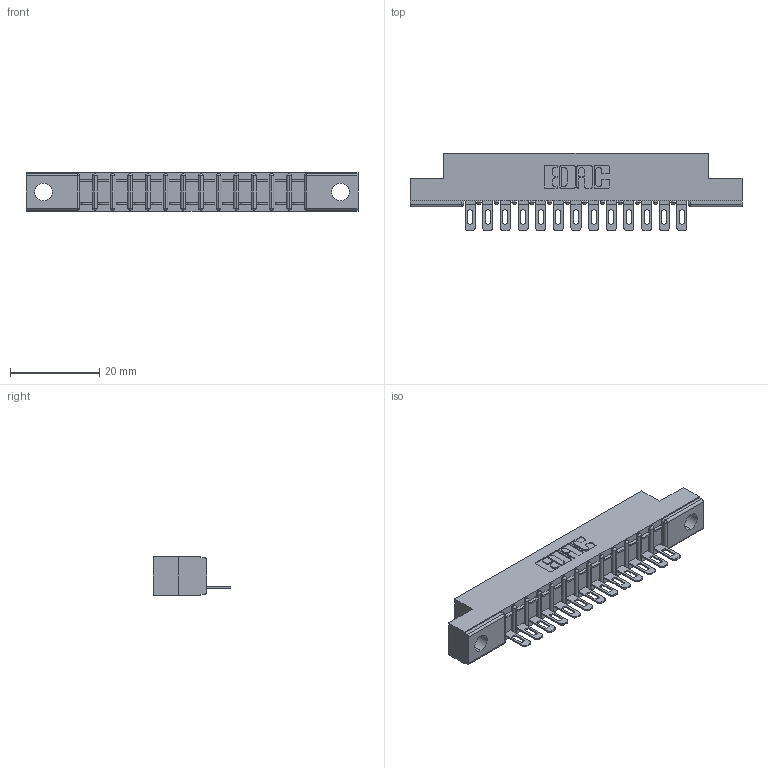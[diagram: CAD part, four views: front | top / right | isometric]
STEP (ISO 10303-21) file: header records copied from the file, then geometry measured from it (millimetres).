
FILE_DESCRIPTION (( 'STEP AP203' ), '1' );
FILE_NAME ('357-013-401-104.STEP', '2020-09-30T14:12:41', ( '' ), ( '' ), 'SwSTEP 2.0', 'SolidWorks 2020', '' );
FILE_SCHEMA (( 'CONFIG_CONTROL_DESIGN' ));
Length unit declared in the file: inch
Products named in the file (3): 357-013-401-104; 307 Part_.156 Dia Mounting Holes; 307-290-002_501
Assembly tree (14 placements, depth 2):
  357-013-401-104
    307 Part_.156 Dia Mounting Holes
    307-290-002_501  x13
Bounding box: 74.52 x 17.42 x 8.71 mm (x, y, z)
Volume: 4820.6 mm3; surface area: 8245.6 mm2
Topology: 14 solids, 14 shells, 1134 faces, 3453 edges, 2262 vertices
Faces by surface type: plane 656, cylinder 450, sphere 28
Entity records: 15932 total; most frequent: CARTESIAN_POINT 2686, ORIENTED_EDGE 2674, DIRECTION 2619, EDGE_CURVE 1337, LINE 1013, VECTOR 1013, VERTEX_POINT 870, AXIS2_PLACEMENT_3D 803
